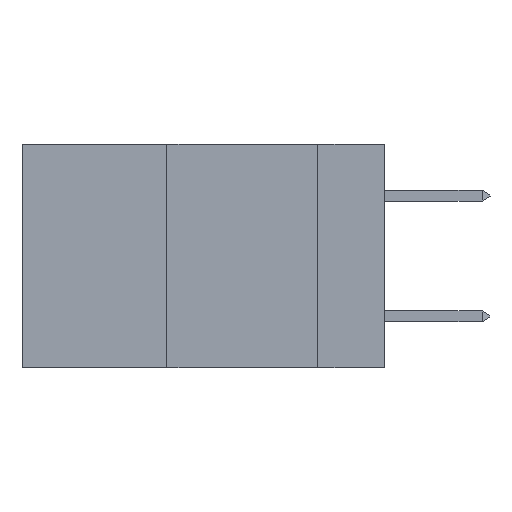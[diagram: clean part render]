
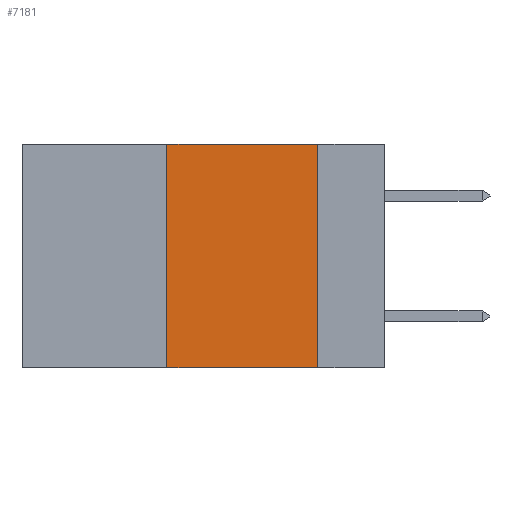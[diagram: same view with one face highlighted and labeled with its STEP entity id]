
A CAD part, left-side view. The second image highlights one B-rep face of the part: STEP entity #7181.
In plain terms, the highlighted planar face has unit normal (-1, 0, 0).
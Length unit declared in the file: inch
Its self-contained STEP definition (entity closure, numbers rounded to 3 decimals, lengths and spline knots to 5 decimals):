
#1971 = CARTESIAN_POINT ( 'NONE',  ( 0., 0.36, 0. ) ) ;
#2159 = DIRECTION ( 'NONE',  ( 0., 0., 1. ) ) ;
#3196 = AXIS2_PLACEMENT_3D ( 'NONE', #5200, #5108, #9228 ) ;
#3265 = VECTOR ( 'NONE', #3483, 39.37008 ) ;
#3294 = CARTESIAN_POINT ( 'NONE',  ( 0., 0.36, -0.37 ) ) ;
#3483 = DIRECTION ( 'NONE',  ( 0., -1., 0. ) ) ;
#3742 = VECTOR ( 'NONE', #13240, 39.37008 ) ;
#4207 = EDGE_CURVE ( 'NONE', #9463, #15728, #15270, .T. ) ;
#4257 = EDGE_CURVE ( 'NONE', #9463, #8308, #14211, .T. ) ;
#4349 = ORIENTED_EDGE ( 'NONE', *, *, #4257, .F. ) ;
#4467 = EDGE_CURVE ( 'NONE', #8308, #6067, #11995, .T. ) ;
#4721 = CARTESIAN_POINT ( 'NONE',  ( 0., 0.6, -0.37 ) ) ;
#5108 = DIRECTION ( 'NONE',  ( 1., 0., 0. ) ) ;
#5167 = EDGE_LOOP ( 'NONE', ( #11761, #6924, #4349, #13022 ) ) ;
#5200 = CARTESIAN_POINT ( 'NONE',  ( 0., 0.6, 0. ) ) ;
#6067 = VERTEX_POINT ( 'NONE', #8589 ) ;
#6292 = LINE ( 'NONE', #17045, #3742 ) ;
#6500 = FACE_OUTER_BOUND ( 'NONE', #5167, .T. ) ;
#6712 = DIRECTION ( 'NONE',  ( 0., -1., 0. ) ) ;
#6924 = ORIENTED_EDGE ( 'NONE', *, *, #4467, .F. ) ;
#6941 = VECTOR ( 'NONE', #6712, 39.37008 ) ;
#7181 = ADVANCED_FACE ( 'NONE', ( #6500 ), #13455, .F. ) ;
#8308 = VERTEX_POINT ( 'NONE', #1971 ) ;
#8589 = CARTESIAN_POINT ( 'NONE',  ( 0., 0.11, 0. ) ) ;
#9228 = DIRECTION ( 'NONE',  ( 0., 0., -1. ) ) ;
#9268 = EDGE_CURVE ( 'NONE', #6067, #15728, #6292, .T. ) ;
#9463 = VERTEX_POINT ( 'NONE', #3294 ) ;
#11299 = CARTESIAN_POINT ( 'NONE',  ( 0., 0.36, 0. ) ) ;
#11761 = ORIENTED_EDGE ( 'NONE', *, *, #9268, .F. ) ;
#11995 = LINE ( 'NONE', #14811, #6941 ) ;
#13022 = ORIENTED_EDGE ( 'NONE', *, *, #4207, .T. ) ;
#13240 = DIRECTION ( 'NONE',  ( 0., 0., -1. ) ) ;
#13455 = PLANE ( 'NONE',  #3196 ) ;
#14211 = LINE ( 'NONE', #11299, #17334 ) ;
#14811 = CARTESIAN_POINT ( 'NONE',  ( 0., 0.6, 0. ) ) ;
#15270 = LINE ( 'NONE', #4721, #3265 ) ;
#15728 = VERTEX_POINT ( 'NONE', #16217 ) ;
#16217 = CARTESIAN_POINT ( 'NONE',  ( 0., 0.11, -0.37 ) ) ;
#17045 = CARTESIAN_POINT ( 'NONE',  ( 0., 0.11, 0. ) ) ;
#17334 = VECTOR ( 'NONE', #2159, 39.37008 ) ;
